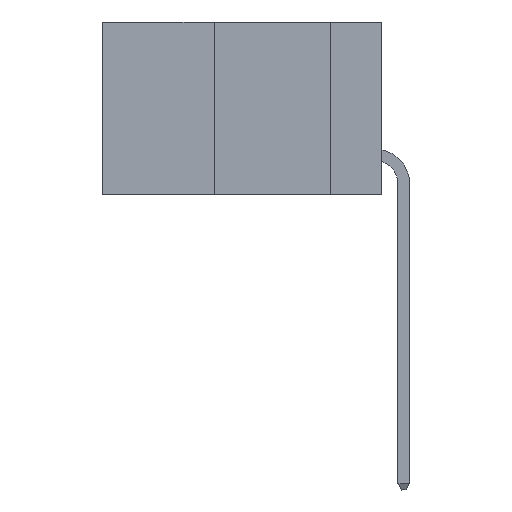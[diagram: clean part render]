
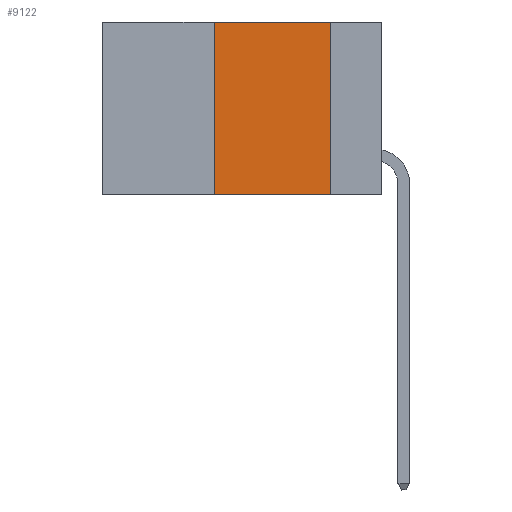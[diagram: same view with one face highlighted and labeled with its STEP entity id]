
A CAD part, left-side view. The second image highlights one B-rep face of the part: STEP entity #9122.
In plain terms, the highlighted planar face has unit normal (-1, 0, 0).
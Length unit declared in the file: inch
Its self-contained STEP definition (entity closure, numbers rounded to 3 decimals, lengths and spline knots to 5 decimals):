
#103 = VECTOR ( 'NONE', #8648, 39.37008 ) ;
#400 = EDGE_CURVE ( 'NONE', #561, #2332, #726, .T. ) ;
#561 = VERTEX_POINT ( 'NONE', #13679 ) ;
#726 = LINE ( 'NONE', #5247, #9843 ) ;
#935 = PLANE ( 'NONE',  #2309 ) ;
#1130 = VERTEX_POINT ( 'NONE', #1340 ) ;
#1240 = DIRECTION ( 'NONE',  ( 1., 0., 0. ) ) ;
#1286 = LINE ( 'NONE', #9328, #16564 ) ;
#1340 = CARTESIAN_POINT ( 'NONE',  ( 0., 0.36, -0.37 ) ) ;
#2309 = AXIS2_PLACEMENT_3D ( 'NONE', #16859, #1240, #6976 ) ;
#2332 = VERTEX_POINT ( 'NONE', #6131 ) ;
#2789 = EDGE_CURVE ( 'NONE', #1130, #2332, #4677, .T. ) ;
#4677 = LINE ( 'NONE', #8863, #15076 ) ;
#5247 = CARTESIAN_POINT ( 'NONE',  ( 0., 0.11, 0. ) ) ;
#6131 = CARTESIAN_POINT ( 'NONE',  ( 0., 0.11, -0.37 ) ) ;
#6252 = ORIENTED_EDGE ( 'NONE', *, *, #2789, .T. ) ;
#6808 = ORIENTED_EDGE ( 'NONE', *, *, #10902, .F. ) ;
#6976 = DIRECTION ( 'NONE',  ( 0., 0., -1. ) ) ;
#7156 = CARTESIAN_POINT ( 'NONE',  ( 0., 0.36, 0. ) ) ;
#7984 = DIRECTION ( 'NONE',  ( 0., -1., 0. ) ) ;
#8648 = DIRECTION ( 'NONE',  ( 0., 0., 1. ) ) ;
#8863 = CARTESIAN_POINT ( 'NONE',  ( 0., 0.6, -0.37 ) ) ;
#9122 = ADVANCED_FACE ( 'NONE', ( #16011 ), #935, .F. ) ;
#9328 = CARTESIAN_POINT ( 'NONE',  ( 0., 0.6, 0. ) ) ;
#9843 = VECTOR ( 'NONE', #16241, 39.37008 ) ;
#10902 = EDGE_CURVE ( 'NONE', #11829, #561, #1286, .T. ) ;
#11598 = DIRECTION ( 'NONE',  ( 0., -1., 0. ) ) ;
#11829 = VERTEX_POINT ( 'NONE', #7156 ) ;
#12699 = CARTESIAN_POINT ( 'NONE',  ( 0., 0.36, 0. ) ) ;
#13594 = EDGE_LOOP ( 'NONE', ( #13596, #6808, #15297, #6252 ) ) ;
#13596 = ORIENTED_EDGE ( 'NONE', *, *, #400, .F. ) ;
#13679 = CARTESIAN_POINT ( 'NONE',  ( 0., 0.11, 0. ) ) ;
#14953 = LINE ( 'NONE', #12699, #103 ) ;
#15076 = VECTOR ( 'NONE', #11598, 39.37008 ) ;
#15297 = ORIENTED_EDGE ( 'NONE', *, *, #16448, .F. ) ;
#16011 = FACE_OUTER_BOUND ( 'NONE', #13594, .T. ) ;
#16241 = DIRECTION ( 'NONE',  ( 0., 0., -1. ) ) ;
#16448 = EDGE_CURVE ( 'NONE', #1130, #11829, #14953, .T. ) ;
#16564 = VECTOR ( 'NONE', #7984, 39.37008 ) ;
#16859 = CARTESIAN_POINT ( 'NONE',  ( 0., 0.6, 0. ) ) ;
